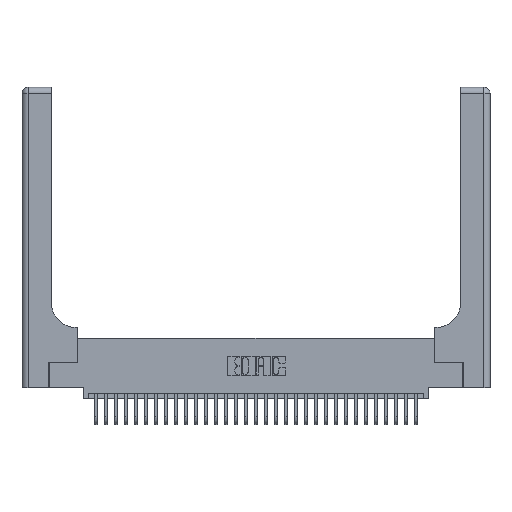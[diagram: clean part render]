
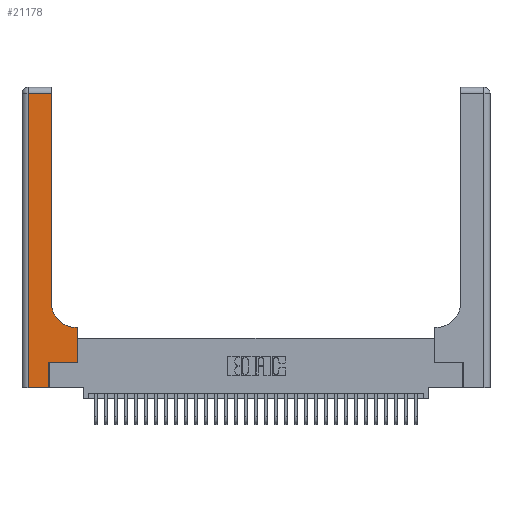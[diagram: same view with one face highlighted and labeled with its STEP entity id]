
A CAD part, top view. The second image highlights one B-rep face of the part: STEP entity #21178.
In plain terms, the highlighted planar face has unit normal (0, 0, 1).
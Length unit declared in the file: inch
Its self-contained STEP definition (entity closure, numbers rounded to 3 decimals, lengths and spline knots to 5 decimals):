
#864 = ORIENTED_EDGE ( 'NONE', *, *, #22743, .T. ) ;
#1280 = ORIENTED_EDGE ( 'NONE', *, *, #28740, .T. ) ;
#1627 = AXIS2_PLACEMENT_3D ( 'NONE', #20168, #4363, #22821 ) ;
#1678 = PLANE ( 'NONE',  #1627 ) ;
#1990 = EDGE_CURVE ( 'NONE', #20330, #26418, #26017, .T. ) ;
#2082 = DIRECTION ( 'NONE',  ( 1., 0., 0. ) ) ;
#2765 = VECTOR ( 'NONE', #2082, 39.37008 ) ;
#3040 = LINE ( 'NONE', #28692, #30221 ) ;
#3215 = LINE ( 'NONE', #30139, #30389 ) ;
#3230 = EDGE_LOOP ( 'NONE', ( #11218, #1280, #15363, #24006, #25662, #20324, #864, #14966, #21972 ) ) ;
#4251 = CARTESIAN_POINT ( 'NONE',  ( 0., 2.94, 0.37 ) ) ;
#4291 = EDGE_CURVE ( 'NONE', #22640, #31288, #15987, .T. ) ;
#4352 = AXIS2_PLACEMENT_3D ( 'NONE', #13206, #31556, #15871 ) ;
#4363 = DIRECTION ( 'NONE',  ( 0., 0., -1. ) ) ;
#5364 = CARTESIAN_POINT ( 'NONE',  ( 0.269, 0.25, 0.37 ) ) ;
#8969 = VECTOR ( 'NONE', #15758, 39.37008 ) ;
#9032 = CARTESIAN_POINT ( 'NONE',  ( 0.2915, 2.94, 0.37 ) ) ;
#9418 = VECTOR ( 'NONE', #31669, 39.37008 ) ;
#9594 = VERTEX_POINT ( 'NONE', #9032 ) ;
#10121 = VECTOR ( 'NONE', #32573, 39.37008 ) ;
#11218 = ORIENTED_EDGE ( 'NONE', *, *, #13334, .T. ) ;
#11305 = CARTESIAN_POINT ( 'NONE',  ( 0.269, 0., 0.37 ) ) ;
#11437 = VERTEX_POINT ( 'NONE', #32913 ) ;
#11579 = CARTESIAN_POINT ( 'NONE',  ( 0.06, 3., 0.37 ) ) ;
#11925 = VERTEX_POINT ( 'NONE', #16394 ) ;
#11990 = DIRECTION ( 'NONE',  ( 0., 1., 0. ) ) ;
#12789 = FACE_OUTER_BOUND ( 'NONE', #3230, .T. ) ;
#13206 = CARTESIAN_POINT ( 'NONE',  ( 0.5415, 0.85, 0.37 ) ) ;
#13334 = EDGE_CURVE ( 'NONE', #26418, #9594, #21524, .T. ) ;
#14966 = ORIENTED_EDGE ( 'NONE', *, *, #17642, .T. ) ;
#15255 = CARTESIAN_POINT ( 'NONE',  ( 0., 0., 0.37 ) ) ;
#15312 = EDGE_CURVE ( 'NONE', #31288, #20472, #16424, .T. ) ;
#15363 = ORIENTED_EDGE ( 'NONE', *, *, #29810, .T. ) ;
#15758 = DIRECTION ( 'NONE',  ( 0., 1., 0. ) ) ;
#15871 = DIRECTION ( 'NONE',  ( 1., 0., 0. ) ) ;
#15987 = LINE ( 'NONE', #23597, #8969 ) ;
#16394 = CARTESIAN_POINT ( 'NONE',  ( 0.06, 2.94, 0.37 ) ) ;
#16424 = LINE ( 'NONE', #5364, #9418 ) ;
#16642 = CARTESIAN_POINT ( 'NONE',  ( 0.5415, 0.6, 0.37 ) ) ;
#16810 = LINE ( 'NONE', #15255, #2765 ) ;
#17121 = LINE ( 'NONE', #11579, #10121 ) ;
#17642 = EDGE_CURVE ( 'NONE', #28263, #20330, #3040, .T. ) ;
#20168 = CARTESIAN_POINT ( 'NONE',  ( 0., 3., 0.37 ) ) ;
#20324 = ORIENTED_EDGE ( 'NONE', *, *, #15312, .T. ) ;
#20330 = VERTEX_POINT ( 'NONE', #16642 ) ;
#20472 = VERTEX_POINT ( 'NONE', #32785 ) ;
#20670 = CARTESIAN_POINT ( 'NONE',  ( 0.5585, 0.6, 0.37 ) ) ;
#20690 = VECTOR ( 'NONE', #29065, 39.37008 ) ;
#21171 = CARTESIAN_POINT ( 'NONE',  ( 0.2915, 3., 0.37 ) ) ;
#21178 = ADVANCED_FACE ( 'NONE', ( #12789 ), #1678, .F. ) ;
#21524 = LINE ( 'NONE', #21171, #20690 ) ;
#21972 = ORIENTED_EDGE ( 'NONE', *, *, #1990, .T. ) ;
#22147 = VECTOR ( 'NONE', #25348, 39.37008 ) ;
#22640 = VERTEX_POINT ( 'NONE', #11305 ) ;
#22743 = EDGE_CURVE ( 'NONE', #20472, #28263, #3215, .T. ) ;
#22821 = DIRECTION ( 'NONE',  ( -1., 0., 0. ) ) ;
#23597 = CARTESIAN_POINT ( 'NONE',  ( 0.269, 0., 0.37 ) ) ;
#23713 = CARTESIAN_POINT ( 'NONE',  ( 0.269, 0.25, 0.37 ) ) ;
#24006 = ORIENTED_EDGE ( 'NONE', *, *, #28218, .T. ) ;
#25348 = DIRECTION ( 'NONE',  ( -1., 0., 0. ) ) ;
#25662 = ORIENTED_EDGE ( 'NONE', *, *, #4291, .T. ) ;
#26017 = CIRCLE ( 'NONE', #4352, 0.25 ) ;
#26418 = VERTEX_POINT ( 'NONE', #28105 ) ;
#28105 = CARTESIAN_POINT ( 'NONE',  ( 0.2915, 0.85, 0.37 ) ) ;
#28218 = EDGE_CURVE ( 'NONE', #11437, #22640, #16810, .T. ) ;
#28263 = VERTEX_POINT ( 'NONE', #20670 ) ;
#28692 = CARTESIAN_POINT ( 'NONE',  ( 0.2915, 0.6, 0.37 ) ) ;
#28740 = EDGE_CURVE ( 'NONE', #9594, #11925, #29099, .T. ) ;
#29065 = DIRECTION ( 'NONE',  ( 0., 1., 0. ) ) ;
#29099 = LINE ( 'NONE', #4251, #22147 ) ;
#29810 = EDGE_CURVE ( 'NONE', #11925, #11437, #17121, .T. ) ;
#30139 = CARTESIAN_POINT ( 'NONE',  ( 0.5585, 0.25, 0.37 ) ) ;
#30221 = VECTOR ( 'NONE', #33916, 39.37008 ) ;
#30389 = VECTOR ( 'NONE', #11990, 39.37008 ) ;
#31288 = VERTEX_POINT ( 'NONE', #23713 ) ;
#31556 = DIRECTION ( 'NONE',  ( 0., 0., -1. ) ) ;
#31669 = DIRECTION ( 'NONE',  ( 1., 0., 0. ) ) ;
#32573 = DIRECTION ( 'NONE',  ( 0., -1., 0. ) ) ;
#32785 = CARTESIAN_POINT ( 'NONE',  ( 0.5585, 0.25, 0.37 ) ) ;
#32913 = CARTESIAN_POINT ( 'NONE',  ( 0.06, 0., 0.37 ) ) ;
#33916 = DIRECTION ( 'NONE',  ( -1., 0., 0. ) ) ;
